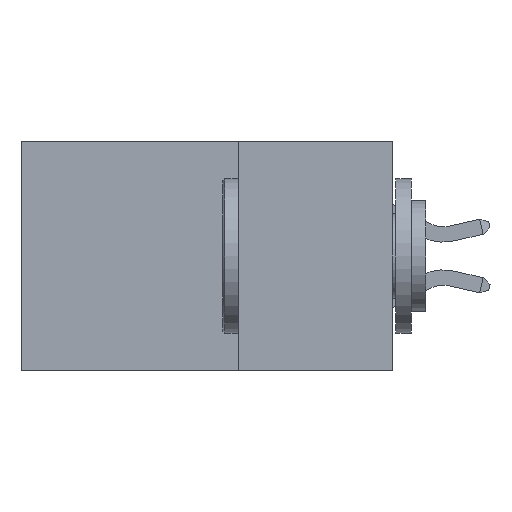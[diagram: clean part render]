
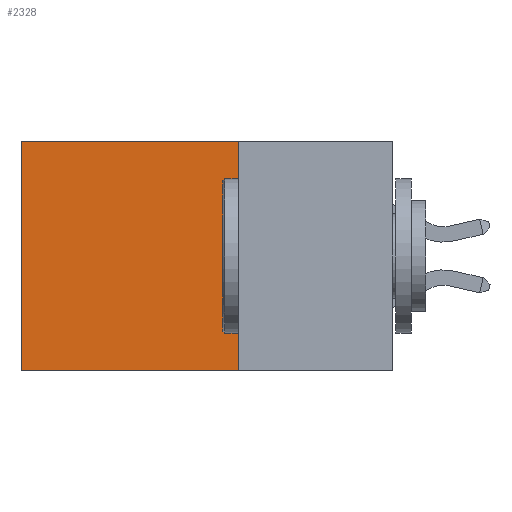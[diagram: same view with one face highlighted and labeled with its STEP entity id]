
A CAD part, left-side view. The second image highlights one B-rep face of the part: STEP entity #2328.
In plain terms, the highlighted planar face has unit normal (-1, 0, 0).
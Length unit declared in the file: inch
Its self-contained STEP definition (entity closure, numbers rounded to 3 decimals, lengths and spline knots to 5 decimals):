
#75 = VERTEX_POINT ( 'NONE', #4457 ) ;
#352 = ORIENTED_EDGE ( 'NONE', *, *, #9775, .F. ) ;
#814 = CARTESIAN_POINT ( 'NONE',  ( 0.2875, 0.25, 0. ) ) ;
#1175 = CARTESIAN_POINT ( 'NONE',  ( 0.2875, 0.25, -0.37 ) ) ;
#1545 = EDGE_CURVE ( 'NONE', #5679, #7176, #5803, .T. ) ;
#1631 = EDGE_LOOP ( 'NONE', ( #3234, #3199, #352, #6438 ) ) ;
#1771 = LINE ( 'NONE', #2174, #9153 ) ;
#2174 = CARTESIAN_POINT ( 'NONE',  ( 0.2875, 0.6, 0. ) ) ;
#2328 = ADVANCED_FACE ( 'NONE', ( #4321 ), #12369, .F. ) ;
#2583 = DIRECTION ( 'NONE',  ( 1., 0., 0. ) ) ;
#2769 = CARTESIAN_POINT ( 'NONE',  ( 0.2875, 0.25, 0. ) ) ;
#3199 = ORIENTED_EDGE ( 'NONE', *, *, #1545, .F. ) ;
#3234 = ORIENTED_EDGE ( 'NONE', *, *, #10370, .T. ) ;
#4113 = VECTOR ( 'NONE', #10381, 39.37008 ) ;
#4321 = FACE_OUTER_BOUND ( 'NONE', #1631, .T. ) ;
#4457 = CARTESIAN_POINT ( 'NONE',  ( 0.2875, 0.6, 0. ) ) ;
#4527 = LINE ( 'NONE', #814, #4113 ) ;
#4897 = CARTESIAN_POINT ( 'NONE',  ( 0.2875, 0.25, 0. ) ) ;
#5063 = CARTESIAN_POINT ( 'NONE',  ( 0.2875, 0.6, -0.37 ) ) ;
#5590 = DIRECTION ( 'NONE',  ( 0., 1., 0. ) ) ;
#5666 = DIRECTION ( 'NONE',  ( 0., 0., -1. ) ) ;
#5679 = VERTEX_POINT ( 'NONE', #10643 ) ;
#5803 = LINE ( 'NONE', #1175, #6389 ) ;
#6041 = AXIS2_PLACEMENT_3D ( 'NONE', #9746, #2583, #7345 ) ;
#6389 = VECTOR ( 'NONE', #5590, 39.37008 ) ;
#6438 = ORIENTED_EDGE ( 'NONE', *, *, #9764, .T. ) ;
#7176 = VERTEX_POINT ( 'NONE', #5063 ) ;
#7345 = DIRECTION ( 'NONE',  ( 0., 0., -1. ) ) ;
#9153 = VECTOR ( 'NONE', #11131, 39.37008 ) ;
#9319 = VECTOR ( 'NONE', #5666, 39.37008 ) ;
#9746 = CARTESIAN_POINT ( 'NONE',  ( 0.2875, 0.25, 0. ) ) ;
#9764 = EDGE_CURVE ( 'NONE', #11387, #75, #4527, .T. ) ;
#9775 = EDGE_CURVE ( 'NONE', #11387, #5679, #11898, .T. ) ;
#10370 = EDGE_CURVE ( 'NONE', #75, #7176, #1771, .T. ) ;
#10381 = DIRECTION ( 'NONE',  ( 0., 1., 0. ) ) ;
#10643 = CARTESIAN_POINT ( 'NONE',  ( 0.2875, 0.25, -0.37 ) ) ;
#11131 = DIRECTION ( 'NONE',  ( 0., 0., -1. ) ) ;
#11387 = VERTEX_POINT ( 'NONE', #4897 ) ;
#11898 = LINE ( 'NONE', #2769, #9319 ) ;
#12369 = PLANE ( 'NONE',  #6041 ) ;
